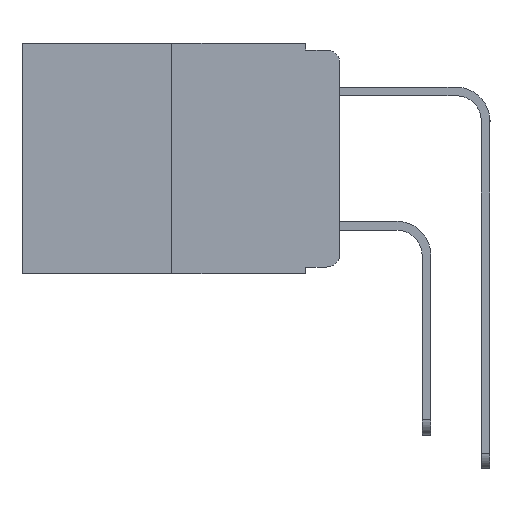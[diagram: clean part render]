
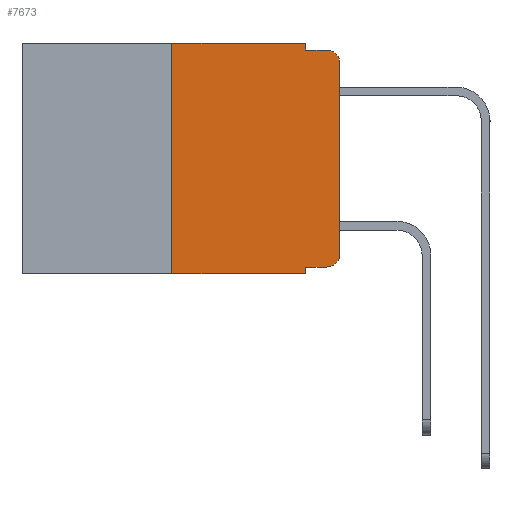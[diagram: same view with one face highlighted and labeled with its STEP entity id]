
A CAD part, left-side view. The second image highlights one B-rep face of the part: STEP entity #7673.
In plain terms, the highlighted planar face has unit normal (-1, 0, 0).
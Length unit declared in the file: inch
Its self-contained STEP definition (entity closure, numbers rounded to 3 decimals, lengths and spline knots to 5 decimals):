
#244 = DIRECTION ( 'NONE',  ( 0., -1., 0. ) ) ;
#436 = ORIENTED_EDGE ( 'NONE', *, *, #14023, .T. ) ;
#453 = VERTEX_POINT ( 'NONE', #16310 ) ;
#462 = VERTEX_POINT ( 'NONE', #10967 ) ;
#909 = LINE ( 'NONE', #13114, #4664 ) ;
#974 = ORIENTED_EDGE ( 'NONE', *, *, #2765, .F. ) ;
#1231 = ORIENTED_EDGE ( 'NONE', *, *, #17592, .F. ) ;
#1410 = PLANE ( 'NONE',  #18403 ) ;
#1438 = EDGE_CURVE ( 'NONE', #453, #21421, #9058, .T. ) ;
#2017 = DIRECTION ( 'NONE',  ( -1., 0., 0. ) ) ;
#2088 = LINE ( 'NONE', #10961, #7534 ) ;
#2107 = LINE ( 'NONE', #18638, #11798 ) ;
#2365 = DIRECTION ( 'NONE',  ( 0., -1., 0. ) ) ;
#2765 = EDGE_CURVE ( 'NONE', #8543, #8163, #909, .T. ) ;
#2778 = CARTESIAN_POINT ( 'NONE',  ( 0., 0.051, -0.333 ) ) ;
#2794 = ORIENTED_EDGE ( 'NONE', *, *, #16802, .T. ) ;
#2993 = VECTOR ( 'NONE', #2365, 39.37008 ) ;
#3287 = DIRECTION ( 'NONE',  ( 0., 0., -1. ) ) ;
#3374 = VECTOR ( 'NONE', #17269, 39.37008 ) ;
#3691 = CARTESIAN_POINT ( 'NONE',  ( 0., 0.02, -0.01 ) ) ;
#4664 = VECTOR ( 'NONE', #244, 39.37008 ) ;
#4774 = FACE_OUTER_BOUND ( 'NONE', #8222, .T. ) ;
#6680 = CARTESIAN_POINT ( 'NONE',  ( 0., 0.051, -0.343 ) ) ;
#6868 = DIRECTION ( 'NONE',  ( -1., 0., 0. ) ) ;
#7534 = VECTOR ( 'NONE', #23409, 39.37008 ) ;
#7673 = ADVANCED_FACE ( 'NONE', ( #4774 ), #1410, .F. ) ;
#7810 = DIRECTION ( 'NONE',  ( 0., -1., 0. ) ) ;
#7867 = LINE ( 'NONE', #18635, #2993 ) ;
#7869 = ORIENTED_EDGE ( 'NONE', *, *, #19968, .F. ) ;
#8163 = VERTEX_POINT ( 'NONE', #15728 ) ;
#8222 = EDGE_LOOP ( 'NONE', ( #12360, #19186, #1231, #7869, #974, #23318, #2794, #10527, #436, #19301 ) ) ;
#8543 = VERTEX_POINT ( 'NONE', #23068 ) ;
#8726 = CARTESIAN_POINT ( 'NONE',  ( 0., 0.25, 0. ) ) ;
#8841 = VECTOR ( 'NONE', #21261, 39.37008 ) ;
#9058 = LINE ( 'NONE', #15416, #12732 ) ;
#9254 = CARTESIAN_POINT ( 'NONE',  ( 0., 0., -0.313 ) ) ;
#9320 = EDGE_CURVE ( 'NONE', #462, #15679, #16053, .T. ) ;
#10325 = CARTESIAN_POINT ( 'NONE',  ( 0., 0.25, -0.343 ) ) ;
#10527 = ORIENTED_EDGE ( 'NONE', *, *, #1438, .F. ) ;
#10961 = CARTESIAN_POINT ( 'NONE',  ( 0., 0.051, 0. ) ) ;
#10967 = CARTESIAN_POINT ( 'NONE',  ( 0., 0., -0.03 ) ) ;
#11552 = CARTESIAN_POINT ( 'NONE',  ( 0., 0.051, -0.01 ) ) ;
#11798 = VECTOR ( 'NONE', #7810, 39.37008 ) ;
#11836 = VECTOR ( 'NONE', #14480, 39.37008 ) ;
#12360 = ORIENTED_EDGE ( 'NONE', *, *, #16609, .T. ) ;
#12653 = CARTESIAN_POINT ( 'NONE',  ( 0., 0., 0. ) ) ;
#12732 = VECTOR ( 'NONE', #17201, 39.37008 ) ;
#12936 = CARTESIAN_POINT ( 'NONE',  ( 0., 0.02, -0.03 ) ) ;
#13114 = CARTESIAN_POINT ( 'NONE',  ( 0., 0.473, 0. ) ) ;
#13544 = EDGE_CURVE ( 'NONE', #17849, #8543, #22551, .T. ) ;
#13618 = LINE ( 'NONE', #2778, #3374 ) ;
#14009 = AXIS2_PLACEMENT_3D ( 'NONE', #17711, #6868, #19518 ) ;
#14023 = EDGE_CURVE ( 'NONE', #453, #16079, #13618, .T. ) ;
#14191 = DIRECTION ( 'NONE',  ( 1., 0., 0. ) ) ;
#14480 = DIRECTION ( 'NONE',  ( 0., 0., 1. ) ) ;
#14619 = VERTEX_POINT ( 'NONE', #11552 ) ;
#14758 = DIRECTION ( 'NONE',  ( 0., 0., -1. ) ) ;
#15077 = VERTEX_POINT ( 'NONE', #9254 ) ;
#15416 = CARTESIAN_POINT ( 'NONE',  ( 0., 0.051, 0. ) ) ;
#15679 = VERTEX_POINT ( 'NONE', #3691 ) ;
#15728 = CARTESIAN_POINT ( 'NONE',  ( 0., 0.051, 0. ) ) ;
#15878 = EDGE_CURVE ( 'NONE', #16079, #15077, #22224, .T. ) ;
#16053 = CIRCLE ( 'NONE', #22415, 0.02 ) ;
#16079 = VERTEX_POINT ( 'NONE', #21898 ) ;
#16310 = CARTESIAN_POINT ( 'NONE',  ( 0., 0.051, -0.333 ) ) ;
#16609 = EDGE_CURVE ( 'NONE', #15077, #462, #21363, .T. ) ;
#16802 = EDGE_CURVE ( 'NONE', #17849, #21421, #7867, .T. ) ;
#17201 = DIRECTION ( 'NONE',  ( 0., 0., -1. ) ) ;
#17269 = DIRECTION ( 'NONE',  ( 0., -1., 0. ) ) ;
#17592 = EDGE_CURVE ( 'NONE', #14619, #15679, #2107, .T. ) ;
#17708 = CARTESIAN_POINT ( 'NONE',  ( 0., 0.473, 0. ) ) ;
#17711 = CARTESIAN_POINT ( 'NONE',  ( 0., 0.02, -0.313 ) ) ;
#17849 = VERTEX_POINT ( 'NONE', #10325 ) ;
#18403 = AXIS2_PLACEMENT_3D ( 'NONE', #17708, #14191, #3287 ) ;
#18635 = CARTESIAN_POINT ( 'NONE',  ( 0., 0.473, -0.343 ) ) ;
#18638 = CARTESIAN_POINT ( 'NONE',  ( 0., 0.051, -0.01 ) ) ;
#19186 = ORIENTED_EDGE ( 'NONE', *, *, #9320, .T. ) ;
#19301 = ORIENTED_EDGE ( 'NONE', *, *, #15878, .T. ) ;
#19518 = DIRECTION ( 'NONE',  ( 0., 0., -1. ) ) ;
#19968 = EDGE_CURVE ( 'NONE', #8163, #14619, #2088, .T. ) ;
#21261 = DIRECTION ( 'NONE',  ( 0., 0., 1. ) ) ;
#21363 = LINE ( 'NONE', #12653, #11836 ) ;
#21421 = VERTEX_POINT ( 'NONE', #6680 ) ;
#21898 = CARTESIAN_POINT ( 'NONE',  ( 0., 0.02, -0.333 ) ) ;
#22224 = CIRCLE ( 'NONE', #14009, 0.02 ) ;
#22415 = AXIS2_PLACEMENT_3D ( 'NONE', #12936, #2017, #14758 ) ;
#22551 = LINE ( 'NONE', #8726, #8841 ) ;
#23068 = CARTESIAN_POINT ( 'NONE',  ( 0., 0.25, 0. ) ) ;
#23318 = ORIENTED_EDGE ( 'NONE', *, *, #13544, .F. ) ;
#23409 = DIRECTION ( 'NONE',  ( 0., 0., -1. ) ) ;
